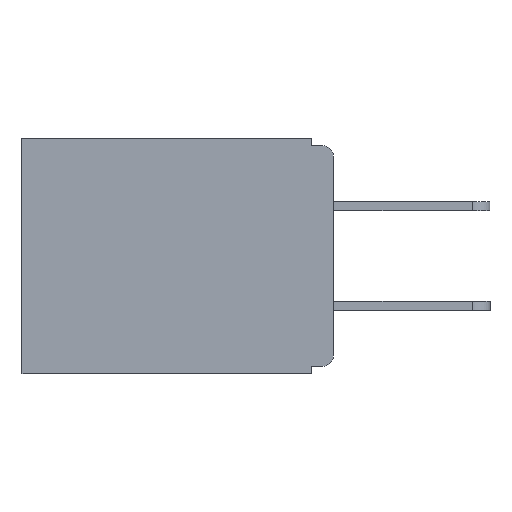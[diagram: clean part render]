
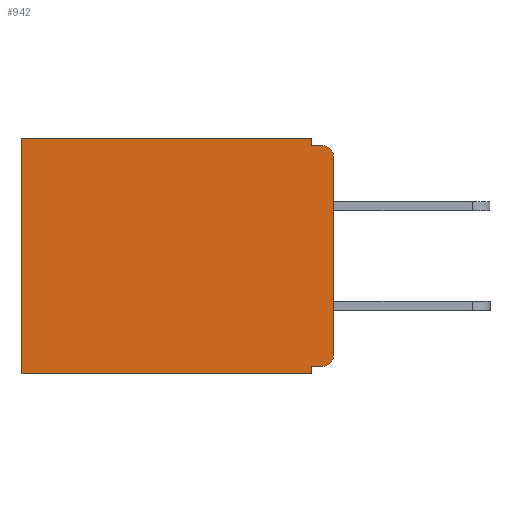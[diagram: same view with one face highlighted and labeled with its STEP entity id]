
A CAD part, left-side view. The second image highlights one B-rep face of the part: STEP entity #942.
In plain terms, the highlighted planar face has unit normal (-1, 0, 0).
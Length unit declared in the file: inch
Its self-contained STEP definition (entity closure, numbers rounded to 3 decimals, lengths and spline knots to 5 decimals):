
#19 = CARTESIAN_POINT ( 'NONE',  ( 0.3, 0., -0.32 ) ) ;
#97 = CARTESIAN_POINT ( 'NONE',  ( 0.3, 0., 0. ) ) ;
#294 = FACE_OUTER_BOUND ( 'NONE', #6678, .T. ) ;
#351 = LINE ( 'NONE', #8959, #10695 ) ;
#401 = DIRECTION ( 'NONE',  ( 0., 0., -1. ) ) ;
#438 = ORIENTED_EDGE ( 'NONE', *, *, #5391, .F. ) ;
#613 = ORIENTED_EDGE ( 'NONE', *, *, #9365, .F. ) ;
#638 = VERTEX_POINT ( 'NONE', #2311 ) ;
#684 = EDGE_CURVE ( 'NONE', #3121, #1340, #8171, .T. ) ;
#759 = VERTEX_POINT ( 'NONE', #4918 ) ;
#845 = VECTOR ( 'NONE', #4493, 39.37008 ) ;
#942 = ADVANCED_FACE ( 'NONE', ( #294 ), #7806, .F. ) ;
#978 = EDGE_CURVE ( 'NONE', #6281, #10249, #4535, .T. ) ;
#1163 = DIRECTION ( 'NONE',  ( 0., 0., -1. ) ) ;
#1310 = DIRECTION ( 'NONE',  ( 0., 1., 0. ) ) ;
#1340 = VERTEX_POINT ( 'NONE', #5767 ) ;
#1458 = AXIS2_PLACEMENT_3D ( 'NONE', #4886, #1664, #7409 ) ;
#1664 = DIRECTION ( 'NONE',  ( -1., 0., 0. ) ) ;
#2190 = VECTOR ( 'NONE', #9871, 39.37008 ) ;
#2311 = CARTESIAN_POINT ( 'NONE',  ( 0.3, 0.031, -0.33 ) ) ;
#2518 = CARTESIAN_POINT ( 'NONE',  ( 0.3, 0.437, -0.33 ) ) ;
#2731 = CARTESIAN_POINT ( 'NONE',  ( 0.3, 0.031, -0.33 ) ) ;
#2736 = VECTOR ( 'NONE', #1310, 39.37008 ) ;
#2743 = ORIENTED_EDGE ( 'NONE', *, *, #4103, .T. ) ;
#2846 = DIRECTION ( 'NONE',  ( 1., 0., 0. ) ) ;
#2854 = LINE ( 'NONE', #4330, #3773 ) ;
#2937 = ORIENTED_EDGE ( 'NONE', *, *, #6737, .F. ) ;
#3121 = VERTEX_POINT ( 'NONE', #5271 ) ;
#3253 = CARTESIAN_POINT ( 'NONE',  ( 0.3, 0.031, 0. ) ) ;
#3773 = VECTOR ( 'NONE', #9248, 39.37008 ) ;
#4048 = VECTOR ( 'NONE', #8285, 39.37008 ) ;
#4103 = EDGE_CURVE ( 'NONE', #4377, #9954, #9855, .T. ) ;
#4330 = CARTESIAN_POINT ( 'NONE',  ( 0.3, 0.031, 0. ) ) ;
#4377 = VERTEX_POINT ( 'NONE', #4620 ) ;
#4493 = DIRECTION ( 'NONE',  ( 0., 0., -1. ) ) ;
#4535 = CIRCLE ( 'NONE', #4968, 0.015 ) ;
#4539 = CARTESIAN_POINT ( 'NONE',  ( 0.3, 0., -0.33 ) ) ;
#4591 = LINE ( 'NONE', #19, #5630 ) ;
#4620 = CARTESIAN_POINT ( 'NONE',  ( 0.3, 0.437, 0. ) ) ;
#4630 = EDGE_CURVE ( 'NONE', #638, #9954, #8953, .T. ) ;
#4886 = CARTESIAN_POINT ( 'NONE',  ( 0.3, 0.015, -0.025 ) ) ;
#4918 = CARTESIAN_POINT ( 'NONE',  ( 0.3, 0.031, -0.32 ) ) ;
#4926 = DIRECTION ( 'NONE',  ( 0., 1., 0. ) ) ;
#4968 = AXIS2_PLACEMENT_3D ( 'NONE', #6088, #8646, #401 ) ;
#5020 = ORIENTED_EDGE ( 'NONE', *, *, #978, .T. ) ;
#5136 = CARTESIAN_POINT ( 'NONE',  ( 0.3, 0., -0.305 ) ) ;
#5186 = CARTESIAN_POINT ( 'NONE',  ( 0.3, 0., -0.33 ) ) ;
#5271 = CARTESIAN_POINT ( 'NONE',  ( 0.3, 0., -0.025 ) ) ;
#5391 = EDGE_CURVE ( 'NONE', #6438, #8017, #2854, .T. ) ;
#5630 = VECTOR ( 'NONE', #4926, 39.37008 ) ;
#5767 = CARTESIAN_POINT ( 'NONE',  ( 0.3, 0.015, -0.01 ) ) ;
#5850 = VECTOR ( 'NONE', #10189, 39.37008 ) ;
#6088 = CARTESIAN_POINT ( 'NONE',  ( 0.3, 0.015, -0.305 ) ) ;
#6263 = AXIS2_PLACEMENT_3D ( 'NONE', #10307, #2846, #1163 ) ;
#6281 = VERTEX_POINT ( 'NONE', #9724 ) ;
#6405 = CARTESIAN_POINT ( 'NONE',  ( 0.3, 0.437, -0.33 ) ) ;
#6438 = VERTEX_POINT ( 'NONE', #3253 ) ;
#6678 = EDGE_LOOP ( 'NONE', ( #7071, #8780, #7829, #438, #7340, #2743, #9870, #613, #2937, #5020 ) ) ;
#6737 = EDGE_CURVE ( 'NONE', #6281, #759, #4591, .T. ) ;
#6995 = EDGE_CURVE ( 'NONE', #8017, #1340, #351, .T. ) ;
#7071 = ORIENTED_EDGE ( 'NONE', *, *, #8411, .F. ) ;
#7340 = ORIENTED_EDGE ( 'NONE', *, *, #10250, .T. ) ;
#7409 = DIRECTION ( 'NONE',  ( 0., 0., -1. ) ) ;
#7806 = PLANE ( 'NONE',  #6263 ) ;
#7829 = ORIENTED_EDGE ( 'NONE', *, *, #6995, .F. ) ;
#8017 = VERTEX_POINT ( 'NONE', #9860 ) ;
#8171 = CIRCLE ( 'NONE', #1458, 0.015 ) ;
#8285 = DIRECTION ( 'NONE',  ( 0., 0., -1. ) ) ;
#8411 = EDGE_CURVE ( 'NONE', #3121, #10249, #9104, .T. ) ;
#8646 = DIRECTION ( 'NONE',  ( -1., 0., 0. ) ) ;
#8780 = ORIENTED_EDGE ( 'NONE', *, *, #684, .T. ) ;
#8953 = LINE ( 'NONE', #4539, #2736 ) ;
#8959 = CARTESIAN_POINT ( 'NONE',  ( 0.3, 0., -0.01 ) ) ;
#8964 = LINE ( 'NONE', #2731, #5850 ) ;
#9104 = LINE ( 'NONE', #5186, #845 ) ;
#9248 = DIRECTION ( 'NONE',  ( 0., 0., -1. ) ) ;
#9365 = EDGE_CURVE ( 'NONE', #759, #638, #8964, .T. ) ;
#9724 = CARTESIAN_POINT ( 'NONE',  ( 0.3, 0.015, -0.32 ) ) ;
#9855 = LINE ( 'NONE', #2518, #4048 ) ;
#9860 = CARTESIAN_POINT ( 'NONE',  ( 0.3, 0.031, -0.01 ) ) ;
#9870 = ORIENTED_EDGE ( 'NONE', *, *, #4630, .F. ) ;
#9871 = DIRECTION ( 'NONE',  ( 0., 1., 0. ) ) ;
#9954 = VERTEX_POINT ( 'NONE', #6405 ) ;
#10052 = LINE ( 'NONE', #97, #2190 ) ;
#10189 = DIRECTION ( 'NONE',  ( 0., 0., -1. ) ) ;
#10249 = VERTEX_POINT ( 'NONE', #5136 ) ;
#10250 = EDGE_CURVE ( 'NONE', #6438, #4377, #10052, .T. ) ;
#10307 = CARTESIAN_POINT ( 'NONE',  ( 0.3, 0., -0.33 ) ) ;
#10556 = DIRECTION ( 'NONE',  ( 0., -1., 0. ) ) ;
#10695 = VECTOR ( 'NONE', #10556, 39.37008 ) ;
